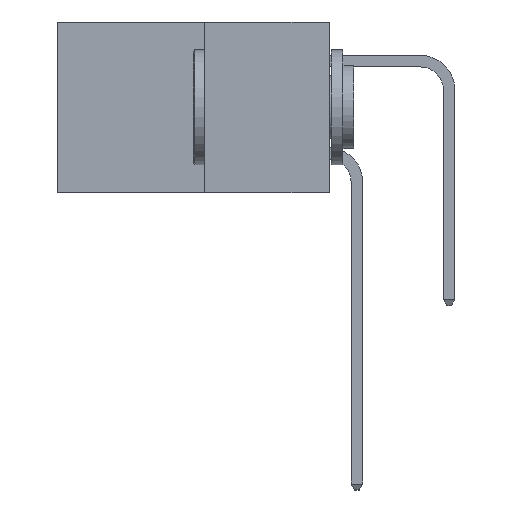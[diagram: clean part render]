
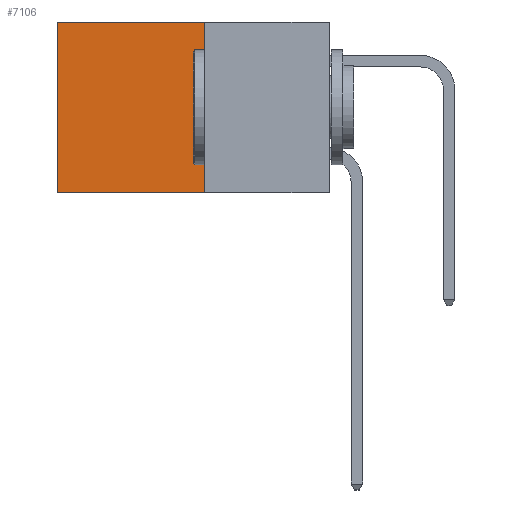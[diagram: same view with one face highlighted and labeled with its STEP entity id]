
A CAD part, left-side view. The second image highlights one B-rep face of the part: STEP entity #7106.
In plain terms, the highlighted planar face has unit normal (-1, 0, 0).
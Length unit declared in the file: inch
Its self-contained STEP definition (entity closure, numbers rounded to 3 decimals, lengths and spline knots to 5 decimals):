
#30 = VECTOR ( 'NONE', #6773, 39.37008 ) ;
#120 = EDGE_CURVE ( 'NONE', #12380, #15102, #483, .T. ) ;
#483 = LINE ( 'NONE', #5931, #30 ) ;
#612 = VERTEX_POINT ( 'NONE', #5947 ) ;
#632 = ORIENTED_EDGE ( 'NONE', *, *, #6439, .T. ) ;
#699 = VERTEX_POINT ( 'NONE', #4584 ) ;
#1528 = VECTOR ( 'NONE', #4431, 39.37008 ) ;
#1989 = LINE ( 'NONE', #4471, #1528 ) ;
#2033 = AXIS2_PLACEMENT_3D ( 'NONE', #4502, #4445, #4340 ) ;
#2198 = VECTOR ( 'NONE', #2259, 39.37008 ) ;
#2259 = DIRECTION ( 'NONE',  ( 0., 0., -1. ) ) ;
#2358 = CARTESIAN_POINT ( 'NONE',  ( 0.277, 0.59, -0.37 ) ) ;
#2879 = ORIENTED_EDGE ( 'NONE', *, *, #15580, .F. ) ;
#3386 = VECTOR ( 'NONE', #6229, 39.37008 ) ;
#3798 = LINE ( 'NONE', #4874, #3386 ) ;
#4340 = DIRECTION ( 'NONE',  ( 0., 0., -1. ) ) ;
#4431 = DIRECTION ( 'NONE',  ( 0., 1., 0. ) ) ;
#4445 = DIRECTION ( 'NONE',  ( 1., 0., 0. ) ) ;
#4471 = CARTESIAN_POINT ( 'NONE',  ( 0.277, 0.27, 0. ) ) ;
#4502 = CARTESIAN_POINT ( 'NONE',  ( 0.277, 0.27, -0.37 ) ) ;
#4581 = PLANE ( 'NONE',  #2033 ) ;
#4584 = CARTESIAN_POINT ( 'NONE',  ( 0.277, 0.59, -0.37 ) ) ;
#4874 = CARTESIAN_POINT ( 'NONE',  ( 0.277, 0.27, -0.37 ) ) ;
#5931 = CARTESIAN_POINT ( 'NONE',  ( 0.277, 0.27, -0.37 ) ) ;
#5947 = CARTESIAN_POINT ( 'NONE',  ( 0.277, 0.59, 0. ) ) ;
#6229 = DIRECTION ( 'NONE',  ( 0., 1., 0. ) ) ;
#6324 = EDGE_CURVE ( 'NONE', #12380, #612, #1989, .T. ) ;
#6439 = EDGE_CURVE ( 'NONE', #612, #699, #9511, .T. ) ;
#6773 = DIRECTION ( 'NONE',  ( 0., 0., -1. ) ) ;
#7106 = ADVANCED_FACE ( 'NONE', ( #12272 ), #4581, .F. ) ;
#7906 = ORIENTED_EDGE ( 'NONE', *, *, #6324, .T. ) ;
#9291 = CARTESIAN_POINT ( 'NONE',  ( 0.277, 0.27, 0. ) ) ;
#9511 = LINE ( 'NONE', #2358, #2198 ) ;
#12272 = FACE_OUTER_BOUND ( 'NONE', #17122, .T. ) ;
#12380 = VERTEX_POINT ( 'NONE', #9291 ) ;
#15102 = VERTEX_POINT ( 'NONE', #16097 ) ;
#15580 = EDGE_CURVE ( 'NONE', #15102, #699, #3798, .T. ) ;
#15965 = ORIENTED_EDGE ( 'NONE', *, *, #120, .F. ) ;
#16097 = CARTESIAN_POINT ( 'NONE',  ( 0.277, 0.27, -0.37 ) ) ;
#17122 = EDGE_LOOP ( 'NONE', ( #632, #2879, #15965, #7906 ) ) ;
